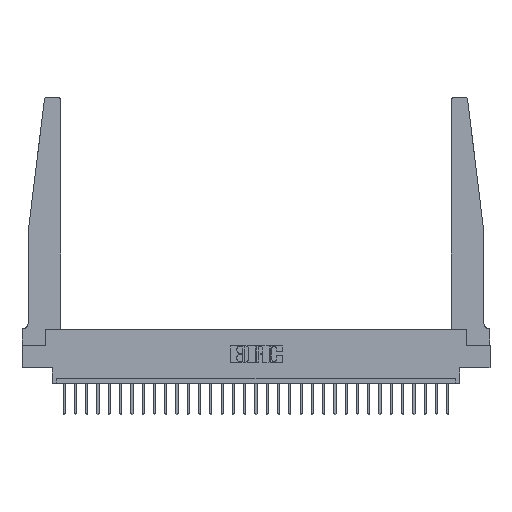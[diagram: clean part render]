
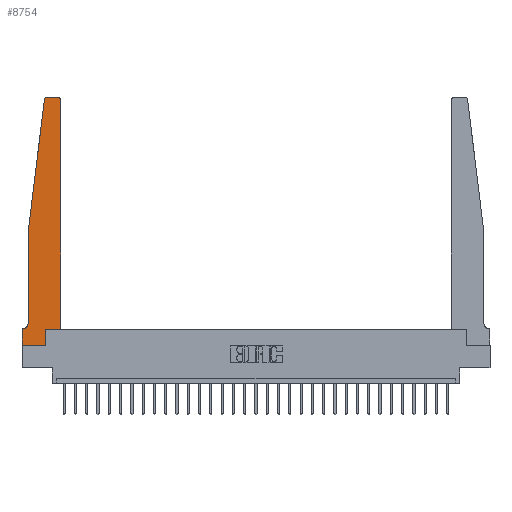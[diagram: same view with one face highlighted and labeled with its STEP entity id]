
A CAD part, top view. The second image highlights one B-rep face of the part: STEP entity #8754.
In plain terms, the highlighted planar face has unit normal (0, 0, 1).
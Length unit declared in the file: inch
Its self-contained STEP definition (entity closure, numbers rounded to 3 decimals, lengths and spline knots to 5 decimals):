
#547 = CARTESIAN_POINT ( 'NONE',  ( 0.065, 1.25, 0.37 ) ) ;
#664 = DIRECTION ( 'NONE',  ( 1., 0., 0. ) ) ;
#936 = CARTESIAN_POINT ( 'NONE',  ( 0., 0., 0.37 ) ) ;
#1358 = DIRECTION ( 'NONE',  ( 0., -1., 0. ) ) ;
#1625 = DIRECTION ( 'NONE',  ( -1., 0., 0. ) ) ;
#1667 = EDGE_CURVE ( 'NONE', #18512, #22535, #11336, .T. ) ;
#2790 = EDGE_CURVE ( 'NONE', #5546, #4798, #10643, .T. ) ;
#3296 = ORIENTED_EDGE ( 'NONE', *, *, #13761, .T. ) ;
#3423 = EDGE_CURVE ( 'NONE', #11136, #20204, #16226, .T. ) ;
#4328 = AXIS2_PLACEMENT_3D ( 'NONE', #20582, #16474, #7458 ) ;
#4459 = CARTESIAN_POINT ( 'NONE',  ( 0.015, 0.2375, 0.37 ) ) ;
#4463 = ORIENTED_EDGE ( 'NONE', *, *, #17709, .T. ) ;
#4478 = ORIENTED_EDGE ( 'NONE', *, *, #21390, .T. ) ;
#4798 = VERTEX_POINT ( 'NONE', #5461 ) ;
#4964 = DIRECTION ( 'NONE',  ( -0.122, -0.992, 0. ) ) ;
#5050 = AXIS2_PLACEMENT_3D ( 'NONE', #9063, #17651, #664 ) ;
#5425 = AXIS2_PLACEMENT_3D ( 'NONE', #4459, #13100, #10995 ) ;
#5461 = CARTESIAN_POINT ( 'NONE',  ( 0.2605, 0., 0.37 ) ) ;
#5546 = VERTEX_POINT ( 'NONE', #936 ) ;
#5782 = LINE ( 'NONE', #20777, #23542 ) ;
#5871 = VECTOR ( 'NONE', #4964, 39.37008 ) ;
#6021 = VERTEX_POINT ( 'NONE', #13946 ) ;
#6163 = VERTEX_POINT ( 'NONE', #16345 ) ;
#6383 = DIRECTION ( 'NONE',  ( 0., 1., 0. ) ) ;
#6500 = DIRECTION ( 'NONE',  ( -1., 0., 0. ) ) ;
#6630 = CARTESIAN_POINT ( 'NONE',  ( 0.25, 2.75, 0.37 ) ) ;
#6754 = LINE ( 'NONE', #19320, #7799 ) ;
#6824 = CARTESIAN_POINT ( 'NONE',  ( 0., 0., 0.37 ) ) ;
#7458 = DIRECTION ( 'NONE',  ( 1., 0., 0. ) ) ;
#7480 = DIRECTION ( 'NONE',  ( 0., 0., 1. ) ) ;
#7799 = VECTOR ( 'NONE', #23601, 39.37008 ) ;
#8328 = VERTEX_POINT ( 'NONE', #13997 ) ;
#8569 = VECTOR ( 'NONE', #6383, 39.37008 ) ;
#8754 = ADVANCED_FACE ( 'NONE', ( #18621 ), #20323, .T. ) ;
#8838 = CARTESIAN_POINT ( 'NONE',  ( 0., 0.1875, 0.37 ) ) ;
#9029 = EDGE_LOOP ( 'NONE', ( #23732, #9719, #10482, #26386, #11423, #16636, #4478, #25556, #4463, #3296, #14769, #16018 ) ) ;
#9063 = CARTESIAN_POINT ( 'NONE',  ( 0.395, 2.72, 0.37 ) ) ;
#9622 = DIRECTION ( 'NONE',  ( 0., 1., 0. ) ) ;
#9719 = ORIENTED_EDGE ( 'NONE', *, *, #11757, .T. ) ;
#10482 = ORIENTED_EDGE ( 'NONE', *, *, #1667, .T. ) ;
#10643 = LINE ( 'NONE', #6824, #25301 ) ;
#10995 = DIRECTION ( 'NONE',  ( -1., 0., 0. ) ) ;
#11136 = VERTEX_POINT ( 'NONE', #17122 ) ;
#11336 = LINE ( 'NONE', #547, #5871 ) ;
#11423 = ORIENTED_EDGE ( 'NONE', *, *, #25986, .T. ) ;
#11594 = CARTESIAN_POINT ( 'NONE',  ( 0.2605, 0.18, 0.37 ) ) ;
#11757 = EDGE_CURVE ( 'NONE', #8328, #18512, #16976, .T. ) ;
#11795 = DIRECTION ( 'NONE',  ( 1., 0., 0. ) ) ;
#11942 = CARTESIAN_POINT ( 'NONE',  ( 0.065, 0.2375, 0.37 ) ) ;
#12896 = DIRECTION ( 'NONE',  ( 1., 0., 0. ) ) ;
#13100 = DIRECTION ( 'NONE',  ( 0., 0., -1. ) ) ;
#13761 = EDGE_CURVE ( 'NONE', #6021, #26555, #22281, .T. ) ;
#13851 = VERTEX_POINT ( 'NONE', #11942 ) ;
#13946 = CARTESIAN_POINT ( 'NONE',  ( 0.2605, 0.18, 0.37 ) ) ;
#13997 = CARTESIAN_POINT ( 'NONE',  ( 0.27653, 2.75, 0.37 ) ) ;
#14545 = CIRCLE ( 'NONE', #5050, 0.03 ) ;
#14769 = ORIENTED_EDGE ( 'NONE', *, *, #17538, .T. ) ;
#15301 = VECTOR ( 'NONE', #6500, 39.37008 ) ;
#16018 = ORIENTED_EDGE ( 'NONE', *, *, #27848, .T. ) ;
#16140 = CARTESIAN_POINT ( 'NONE',  ( 0.425, 0.18, 0.37 ) ) ;
#16226 = LINE ( 'NONE', #24880, #18546 ) ;
#16309 = CARTESIAN_POINT ( 'NONE',  ( 0.425, 0.18, 0.37 ) ) ;
#16345 = CARTESIAN_POINT ( 'NONE',  ( 0.425, 2.72, 0.37 ) ) ;
#16378 = AXIS2_PLACEMENT_3D ( 'NONE', #25020, #7480, #22889 ) ;
#16474 = DIRECTION ( 'NONE',  ( 0., 0., 1. ) ) ;
#16636 = ORIENTED_EDGE ( 'NONE', *, *, #3423, .T. ) ;
#16976 = CIRCLE ( 'NONE', #4328, 0.03 ) ;
#17122 = CARTESIAN_POINT ( 'NONE',  ( 0.015, 0.1875, 0.37 ) ) ;
#17538 = EDGE_CURVE ( 'NONE', #26555, #6163, #26052, .T. ) ;
#17651 = DIRECTION ( 'NONE',  ( 0., 0., 1. ) ) ;
#17709 = EDGE_CURVE ( 'NONE', #4798, #6021, #22069, .T. ) ;
#18512 = VERTEX_POINT ( 'NONE', #24517 ) ;
#18546 = VECTOR ( 'NONE', #1625, 39.37008 ) ;
#18621 = FACE_OUTER_BOUND ( 'NONE', #9029, .T. ) ;
#19063 = LINE ( 'NONE', #6630, #15301 ) ;
#19320 = CARTESIAN_POINT ( 'NONE',  ( 0., 0., 0.37 ) ) ;
#20204 = VERTEX_POINT ( 'NONE', #8838 ) ;
#20323 = PLANE ( 'NONE',  #16378 ) ;
#20429 = CARTESIAN_POINT ( 'NONE',  ( 0.065, 1.25, 0.37 ) ) ;
#20508 = EDGE_CURVE ( 'NONE', #22535, #13851, #5782, .T. ) ;
#20582 = CARTESIAN_POINT ( 'NONE',  ( 0.27653, 2.72, 0.37 ) ) ;
#20777 = CARTESIAN_POINT ( 'NONE',  ( 0.065, 1.25, 0.37 ) ) ;
#21390 = EDGE_CURVE ( 'NONE', #20204, #5546, #6754, .T. ) ;
#21666 = VECTOR ( 'NONE', #9622, 39.37008 ) ;
#22069 = LINE ( 'NONE', #11594, #21666 ) ;
#22281 = LINE ( 'NONE', #16309, #23851 ) ;
#22453 = CARTESIAN_POINT ( 'NONE',  ( 0.395, 2.75, 0.37 ) ) ;
#22535 = VERTEX_POINT ( 'NONE', #20429 ) ;
#22889 = DIRECTION ( 'NONE',  ( 1., 0., 0. ) ) ;
#23078 = CIRCLE ( 'NONE', #5425, 0.05 ) ;
#23542 = VECTOR ( 'NONE', #1358, 39.37008 ) ;
#23601 = DIRECTION ( 'NONE',  ( 0., -1., 0. ) ) ;
#23732 = ORIENTED_EDGE ( 'NONE', *, *, #24331, .T. ) ;
#23851 = VECTOR ( 'NONE', #11795, 39.37008 ) ;
#24331 = EDGE_CURVE ( 'NONE', #24508, #8328, #19063, .T. ) ;
#24508 = VERTEX_POINT ( 'NONE', #22453 ) ;
#24517 = CARTESIAN_POINT ( 'NONE',  ( 0.24675, 2.72367, 0.37 ) ) ;
#24880 = CARTESIAN_POINT ( 'NONE',  ( 0.065, 0.1875, 0.37 ) ) ;
#25020 = CARTESIAN_POINT ( 'NONE',  ( 0., 0.1875, 0.37 ) ) ;
#25301 = VECTOR ( 'NONE', #12896, 39.37008 ) ;
#25556 = ORIENTED_EDGE ( 'NONE', *, *, #2790, .T. ) ;
#25771 = CARTESIAN_POINT ( 'NONE',  ( 0.425, 0.18, 0.37 ) ) ;
#25986 = EDGE_CURVE ( 'NONE', #13851, #11136, #23078, .T. ) ;
#26052 = LINE ( 'NONE', #25771, #8569 ) ;
#26386 = ORIENTED_EDGE ( 'NONE', *, *, #20508, .T. ) ;
#26555 = VERTEX_POINT ( 'NONE', #16140 ) ;
#27848 = EDGE_CURVE ( 'NONE', #6163, #24508, #14545, .T. ) ;
